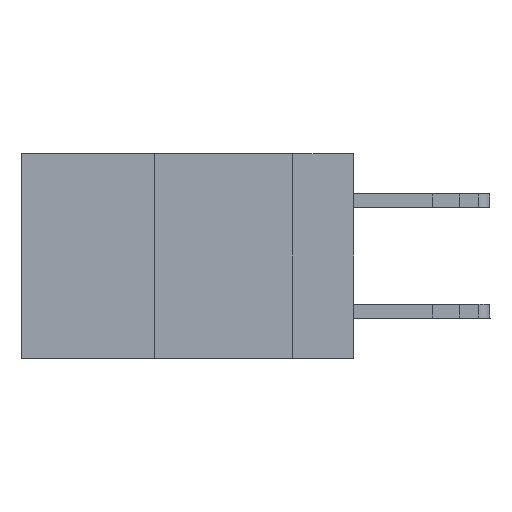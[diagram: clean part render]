
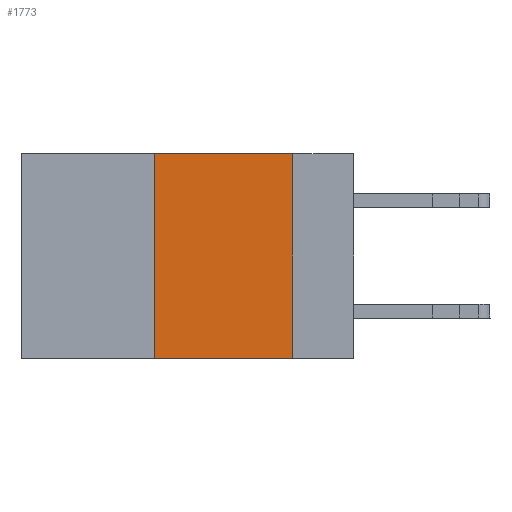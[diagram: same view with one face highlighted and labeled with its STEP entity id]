
A CAD part, left-side view. The second image highlights one B-rep face of the part: STEP entity #1773.
In plain terms, the highlighted planar face has unit normal (-1, 0, 0).
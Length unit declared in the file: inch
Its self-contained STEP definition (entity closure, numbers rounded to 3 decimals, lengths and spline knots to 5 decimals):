
#580 = EDGE_CURVE ( 'NONE', #26074, #7163, #1809, .T. ) ;
#900 = LINE ( 'NONE', #13527, #27371 ) ;
#1773 = ADVANCED_FACE ( 'NONE', ( #26204 ), #8595, .F. ) ;
#1809 = LINE ( 'NONE', #20666, #22242 ) ;
#2392 = LINE ( 'NONE', #25798, #9774 ) ;
#4451 = DIRECTION ( 'NONE',  ( 1., 0., 0. ) ) ;
#5144 = AXIS2_PLACEMENT_3D ( 'NONE', #12800, #4451, #6626 ) ;
#6626 = DIRECTION ( 'NONE',  ( 0., 0., -1. ) ) ;
#7000 = CARTESIAN_POINT ( 'NONE',  ( 0., 0.36, 0. ) ) ;
#7163 = VERTEX_POINT ( 'NONE', #23441 ) ;
#8595 = PLANE ( 'NONE',  #5144 ) ;
#8745 = EDGE_CURVE ( 'NONE', #14054, #21203, #900, .T. ) ;
#9472 = EDGE_CURVE ( 'NONE', #26074, #14054, #9952, .T. ) ;
#9774 = VECTOR ( 'NONE', #23843, 39.37008 ) ;
#9952 = LINE ( 'NONE', #14799, #15312 ) ;
#10215 = DIRECTION ( 'NONE',  ( 0., -1., 0. ) ) ;
#12800 = CARTESIAN_POINT ( 'NONE',  ( 0., 0.6, 0. ) ) ;
#13509 = ORIENTED_EDGE ( 'NONE', *, *, #580, .T. ) ;
#13527 = CARTESIAN_POINT ( 'NONE',  ( 0., 0.6, 0. ) ) ;
#14054 = VERTEX_POINT ( 'NONE', #7000 ) ;
#14574 = CARTESIAN_POINT ( 'NONE',  ( 0., 0.11, 0. ) ) ;
#14799 = CARTESIAN_POINT ( 'NONE',  ( 0., 0.36, 0. ) ) ;
#14983 = DIRECTION ( 'NONE',  ( 0., 0., 1. ) ) ;
#15312 = VECTOR ( 'NONE', #14983, 39.37008 ) ;
#17527 = ORIENTED_EDGE ( 'NONE', *, *, #19467, .F. ) ;
#19239 = ORIENTED_EDGE ( 'NONE', *, *, #9472, .F. ) ;
#19467 = EDGE_CURVE ( 'NONE', #21203, #7163, #2392, .T. ) ;
#20472 = ORIENTED_EDGE ( 'NONE', *, *, #8745, .F. ) ;
#20666 = CARTESIAN_POINT ( 'NONE',  ( 0., 0.6, -0.37 ) ) ;
#21045 = EDGE_LOOP ( 'NONE', ( #17527, #20472, #19239, #13509 ) ) ;
#21203 = VERTEX_POINT ( 'NONE', #14574 ) ;
#22128 = DIRECTION ( 'NONE',  ( 0., -1., 0. ) ) ;
#22242 = VECTOR ( 'NONE', #10215, 39.37008 ) ;
#23441 = CARTESIAN_POINT ( 'NONE',  ( 0., 0.11, -0.37 ) ) ;
#23843 = DIRECTION ( 'NONE',  ( 0., 0., -1. ) ) ;
#25798 = CARTESIAN_POINT ( 'NONE',  ( 0., 0.11, 0. ) ) ;
#26074 = VERTEX_POINT ( 'NONE', #26564 ) ;
#26204 = FACE_OUTER_BOUND ( 'NONE', #21045, .T. ) ;
#26564 = CARTESIAN_POINT ( 'NONE',  ( 0., 0.36, -0.37 ) ) ;
#27371 = VECTOR ( 'NONE', #22128, 39.37008 ) ;
